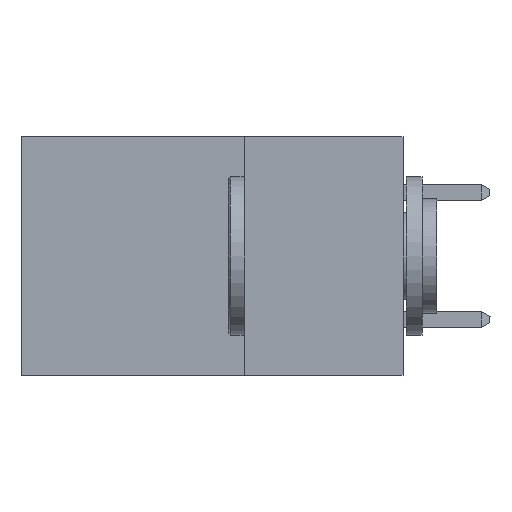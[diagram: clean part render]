
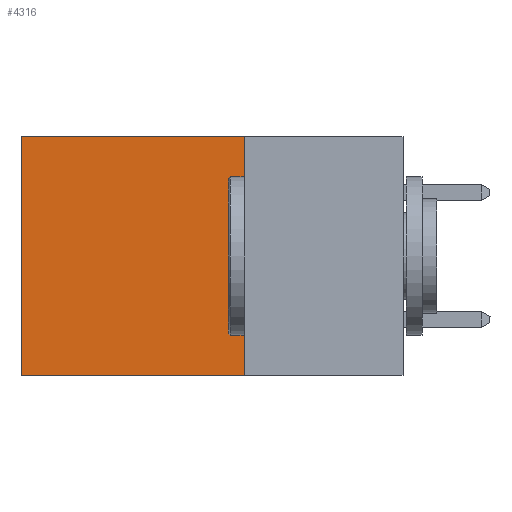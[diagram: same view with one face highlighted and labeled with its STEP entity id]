
A CAD part, left-side view. The second image highlights one B-rep face of the part: STEP entity #4316.
In plain terms, the highlighted planar face has unit normal (-1, 0, 0).
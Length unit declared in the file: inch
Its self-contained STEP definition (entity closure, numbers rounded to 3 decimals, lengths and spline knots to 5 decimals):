
#461 = VECTOR ( 'NONE', #3012, 39.37008 ) ;
#662 = VERTEX_POINT ( 'NONE', #10703 ) ;
#856 = LINE ( 'NONE', #937, #8231 ) ;
#937 = CARTESIAN_POINT ( 'NONE',  ( 0.2875, 0.25, 0. ) ) ;
#1045 = DIRECTION ( 'NONE',  ( 0., 0., -1. ) ) ;
#1503 = EDGE_CURVE ( 'NONE', #12558, #1647, #13380, .T. ) ;
#1647 = VERTEX_POINT ( 'NONE', #8488 ) ;
#2336 = EDGE_LOOP ( 'NONE', ( #3785, #9120, #3980, #3154 ) ) ;
#2376 = CARTESIAN_POINT ( 'NONE',  ( 0.2875, 0.25, -0.375 ) ) ;
#2381 = DIRECTION ( 'NONE',  ( 1., 0., 0. ) ) ;
#3012 = DIRECTION ( 'NONE',  ( 0., 0., -1. ) ) ;
#3154 = ORIENTED_EDGE ( 'NONE', *, *, #13381, .T. ) ;
#3375 = FACE_OUTER_BOUND ( 'NONE', #2336, .T. ) ;
#3471 = VERTEX_POINT ( 'NONE', #9498 ) ;
#3785 = ORIENTED_EDGE ( 'NONE', *, *, #4544, .T. ) ;
#3916 = CARTESIAN_POINT ( 'NONE',  ( 0.2875, 0.6, -0.375 ) ) ;
#3980 = ORIENTED_EDGE ( 'NONE', *, *, #14697, .F. ) ;
#4316 = ADVANCED_FACE ( 'NONE', ( #3375 ), #5991, .F. ) ;
#4392 = LINE ( 'NONE', #15634, #461 ) ;
#4544 = EDGE_CURVE ( 'NONE', #3471, #1647, #11925, .T. ) ;
#5124 = AXIS2_PLACEMENT_3D ( 'NONE', #14993, #2381, #1045 ) ;
#5991 = PLANE ( 'NONE',  #5124 ) ;
#6156 = VECTOR ( 'NONE', #7498, 39.37008 ) ;
#6533 = DIRECTION ( 'NONE',  ( 0., 1., 0. ) ) ;
#6561 = CARTESIAN_POINT ( 'NONE',  ( 0.2875, 0.25, -0.375 ) ) ;
#7498 = DIRECTION ( 'NONE',  ( 0., 0., -1. ) ) ;
#8231 = VECTOR ( 'NONE', #13655, 39.37008 ) ;
#8488 = CARTESIAN_POINT ( 'NONE',  ( 0.2875, 0.6, -0.375 ) ) ;
#9120 = ORIENTED_EDGE ( 'NONE', *, *, #1503, .F. ) ;
#9498 = CARTESIAN_POINT ( 'NONE',  ( 0.2875, 0.6, 0. ) ) ;
#10703 = CARTESIAN_POINT ( 'NONE',  ( 0.2875, 0.25, 0. ) ) ;
#10832 = VECTOR ( 'NONE', #6533, 39.37008 ) ;
#11925 = LINE ( 'NONE', #3916, #6156 ) ;
#12558 = VERTEX_POINT ( 'NONE', #6561 ) ;
#13380 = LINE ( 'NONE', #2376, #10832 ) ;
#13381 = EDGE_CURVE ( 'NONE', #662, #3471, #856, .T. ) ;
#13655 = DIRECTION ( 'NONE',  ( 0., 1., 0. ) ) ;
#14697 = EDGE_CURVE ( 'NONE', #662, #12558, #4392, .T. ) ;
#14993 = CARTESIAN_POINT ( 'NONE',  ( 0.2875, 0.25, -0.375 ) ) ;
#15634 = CARTESIAN_POINT ( 'NONE',  ( 0.2875, 0.25, -0.375 ) ) ;
